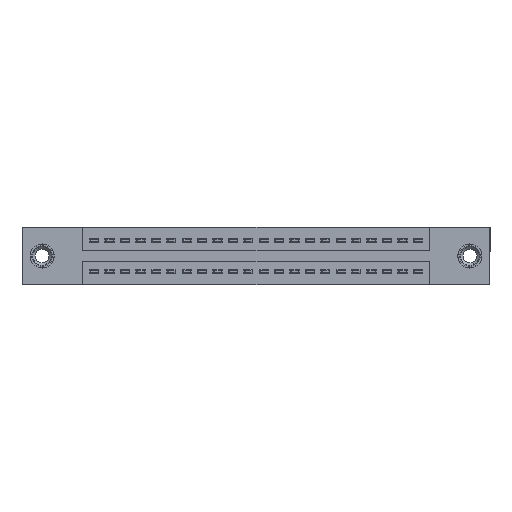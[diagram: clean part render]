
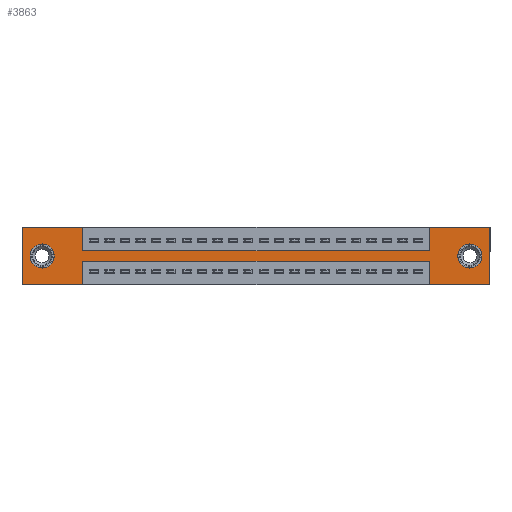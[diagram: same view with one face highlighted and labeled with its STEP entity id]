
A CAD part, front view. The second image highlights one B-rep face of the part: STEP entity #3863.
In plain terms, the highlighted planar face has unit normal (0, -1, 0).
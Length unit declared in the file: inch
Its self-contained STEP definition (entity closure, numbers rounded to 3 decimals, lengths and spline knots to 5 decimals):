
#450 = ORIENTED_EDGE ( 'NONE', *, *, #12869, .T. ) ;
#451 = DIRECTION ( 'NONE',  ( 0., 0., 1. ) ) ;
#697 = DIRECTION ( 'NONE',  ( 0., 0., -1. ) ) ;
#717 = AXIS2_PLACEMENT_3D ( 'NONE', #17985, #14445, #5999 ) ;
#838 = EDGE_CURVE ( 'NONE', #7861, #16075, #21256, .T. ) ;
#957 = DIRECTION ( 'NONE',  ( 1., 0., 0. ) ) ;
#1000 = EDGE_CURVE ( 'NONE', #19194, #17396, #4500, .T. ) ;
#1009 = LINE ( 'NONE', #6715, #16148 ) ;
#1046 = AXIS2_PLACEMENT_3D ( 'NONE', #6978, #21012, #697 ) ;
#1279 = VECTOR ( 'NONE', #3150, 39.37008 ) ;
#1291 = CARTESIAN_POINT ( 'NONE',  ( 2.6425, 0., 0. ) ) ;
#1867 = VERTEX_POINT ( 'NONE', #8113 ) ;
#2496 = EDGE_CURVE ( 'NONE', #21673, #8818, #1009, .T. ) ;
#2686 = DIRECTION ( 'NONE',  ( 0., 0., 1. ) ) ;
#2792 = VERTEX_POINT ( 'NONE', #11082 ) ;
#2934 = CARTESIAN_POINT ( 'NONE',  ( 0., 0., 0. ) ) ;
#2990 = CARTESIAN_POINT ( 'NONE',  ( 0.3925, 0., -0.22 ) ) ;
#3042 = DIRECTION ( 'NONE',  ( 0., 1., 0. ) ) ;
#3150 = DIRECTION ( 'NONE',  ( 1., 0., 0. ) ) ;
#3198 = VECTOR ( 'NONE', #8147, 39.37008 ) ;
#3420 = VERTEX_POINT ( 'NONE', #20329 ) ;
#3492 = VERTEX_POINT ( 'NONE', #18087 ) ;
#3514 = ORIENTED_EDGE ( 'NONE', *, *, #14309, .F. ) ;
#3753 = CARTESIAN_POINT ( 'NONE',  ( 0.13, 0., -0.185 ) ) ;
#3807 = CARTESIAN_POINT ( 'NONE',  ( 0., 0., -0.37 ) ) ;
#3863 = ADVANCED_FACE ( 'NONE', ( #10494, #9686, #5948 ), #14622, .T. ) ;
#4062 = VERTEX_POINT ( 'NONE', #17264 ) ;
#4108 = EDGE_CURVE ( 'NONE', #17717, #3492, #16592, .T. ) ;
#4135 = LINE ( 'NONE', #7260, #18784 ) ;
#4254 = DIRECTION ( 'NONE',  ( 0., 0., 1. ) ) ;
#4474 = DIRECTION ( 'NONE',  ( 0., 0., -1. ) ) ;
#4500 = LINE ( 'NONE', #1291, #3198 ) ;
#5116 = ORIENTED_EDGE ( 'NONE', *, *, #6029, .F. ) ;
#5344 = ORIENTED_EDGE ( 'NONE', *, *, #2496, .F. ) ;
#5537 = ORIENTED_EDGE ( 'NONE', *, *, #838, .F. ) ;
#5947 = VECTOR ( 'NONE', #4254, 39.37008 ) ;
#5948 = FACE_OUTER_BOUND ( 'NONE', #17070, .T. ) ;
#5999 = DIRECTION ( 'NONE',  ( 0., 0., 1. ) ) ;
#6029 = EDGE_CURVE ( 'NONE', #18850, #2792, #16251, .T. ) ;
#6118 = DIRECTION ( 'NONE',  ( 0., -1., 0. ) ) ;
#6328 = VECTOR ( 'NONE', #8868, 39.37008 ) ;
#6452 = DIRECTION ( 'NONE',  ( 0., 0., -1. ) ) ;
#6715 = CARTESIAN_POINT ( 'NONE',  ( 0.3925, 0., -0.22 ) ) ;
#6872 = EDGE_CURVE ( 'NONE', #15528, #1867, #12250, .T. ) ;
#6967 = DIRECTION ( 'NONE',  ( 0., 0., -1. ) ) ;
#6978 = CARTESIAN_POINT ( 'NONE',  ( 2.905, 0., -0.185 ) ) ;
#7174 = CARTESIAN_POINT ( 'NONE',  ( 0.3925, 0., -0.15 ) ) ;
#7260 = CARTESIAN_POINT ( 'NONE',  ( 2.6425, 0., -0.37 ) ) ;
#7368 = LINE ( 'NONE', #17730, #6328 ) ;
#7513 = CARTESIAN_POINT ( 'NONE',  ( 0., 0., 0. ) ) ;
#7577 = CIRCLE ( 'NONE', #1046, 0.078 ) ;
#7738 = EDGE_CURVE ( 'NONE', #17396, #18850, #7368, .T. ) ;
#7777 = EDGE_LOOP ( 'NONE', ( #15441, #13255 ) ) ;
#7861 = VERTEX_POINT ( 'NONE', #15959 ) ;
#7995 = EDGE_CURVE ( 'NONE', #3420, #7861, #19632, .T. ) ;
#8113 = CARTESIAN_POINT ( 'NONE',  ( 0.13, 0., -0.107 ) ) ;
#8147 = DIRECTION ( 'NONE',  ( 0., 0., 1. ) ) ;
#8208 = VECTOR ( 'NONE', #10220, 39.37008 ) ;
#8230 = CARTESIAN_POINT ( 'NONE',  ( 2.6425, 0., 0. ) ) ;
#8436 = CARTESIAN_POINT ( 'NONE',  ( 2.905, 0., -0.263 ) ) ;
#8455 = DIRECTION ( 'NONE',  ( -1., 0., 0. ) ) ;
#8530 = ORIENTED_EDGE ( 'NONE', *, *, #7995, .F. ) ;
#8642 = VECTOR ( 'NONE', #12900, 39.37008 ) ;
#8693 = AXIS2_PLACEMENT_3D ( 'NONE', #3753, #15662, #451 ) ;
#8818 = VERTEX_POINT ( 'NONE', #2990 ) ;
#8868 = DIRECTION ( 'NONE',  ( 1., 0., 0. ) ) ;
#8980 = VERTEX_POINT ( 'NONE', #8436 ) ;
#9023 = VECTOR ( 'NONE', #6967, 39.37008 ) ;
#9129 = EDGE_CURVE ( 'NONE', #8818, #17717, #9462, .T. ) ;
#9171 = CARTESIAN_POINT ( 'NONE',  ( 2.905, 0., -0.107 ) ) ;
#9462 = LINE ( 'NONE', #19499, #8642 ) ;
#9533 = ORIENTED_EDGE ( 'NONE', *, *, #9129, .F. ) ;
#9686 = FACE_BOUND ( 'NONE', #14235, .T. ) ;
#10138 = CARTESIAN_POINT ( 'NONE',  ( 0.3925, 0., 0. ) ) ;
#10220 = DIRECTION ( 'NONE',  ( 0., 0., -1. ) ) ;
#10453 = ORIENTED_EDGE ( 'NONE', *, *, #4108, .F. ) ;
#10494 = FACE_BOUND ( 'NONE', #7777, .T. ) ;
#10948 = CARTESIAN_POINT ( 'NONE',  ( 0.3925, 0., -0.15 ) ) ;
#11082 = CARTESIAN_POINT ( 'NONE',  ( 3.035, 0., -0.37 ) ) ;
#11268 = ORIENTED_EDGE ( 'NONE', *, *, #7738, .F. ) ;
#11320 = CARTESIAN_POINT ( 'NONE',  ( 0., 0., -0.37 ) ) ;
#11463 = ORIENTED_EDGE ( 'NONE', *, *, #17639, .F. ) ;
#11595 = CARTESIAN_POINT ( 'NONE',  ( 0., 0., -0.37 ) ) ;
#12250 = CIRCLE ( 'NONE', #8693, 0.078 ) ;
#12554 = AXIS2_PLACEMENT_3D ( 'NONE', #11320, #6118, #4474 ) ;
#12603 = EDGE_CURVE ( 'NONE', #16075, #19194, #20177, .T. ) ;
#12869 = EDGE_CURVE ( 'NONE', #1867, #15528, #15147, .T. ) ;
#12900 = DIRECTION ( 'NONE',  ( 0., 0., -1. ) ) ;
#13239 = CARTESIAN_POINT ( 'NONE',  ( 2.905, 0., -0.185 ) ) ;
#13255 = ORIENTED_EDGE ( 'NONE', *, *, #16276, .T. ) ;
#14235 = EDGE_LOOP ( 'NONE', ( #450, #20713 ) ) ;
#14309 = EDGE_CURVE ( 'NONE', #4062, #21673, #4135, .T. ) ;
#14445 = DIRECTION ( 'NONE',  ( 0., 1., 0. ) ) ;
#14622 = PLANE ( 'NONE',  #12554 ) ;
#14946 = CARTESIAN_POINT ( 'NONE',  ( 3.035, 0., 0. ) ) ;
#15147 = CIRCLE ( 'NONE', #717, 0.078 ) ;
#15441 = ORIENTED_EDGE ( 'NONE', *, *, #16992, .T. ) ;
#15481 = CARTESIAN_POINT ( 'NONE',  ( 3.035, 0., 0. ) ) ;
#15528 = VERTEX_POINT ( 'NONE', #16933 ) ;
#15662 = DIRECTION ( 'NONE',  ( 0., 1., 0. ) ) ;
#15959 = CARTESIAN_POINT ( 'NONE',  ( 0.3925, 0., 0. ) ) ;
#16075 = VERTEX_POINT ( 'NONE', #7174 ) ;
#16148 = VECTOR ( 'NONE', #8455, 39.37008 ) ;
#16206 = VECTOR ( 'NONE', #957, 39.37008 ) ;
#16251 = LINE ( 'NONE', #15481, #9023 ) ;
#16276 = EDGE_CURVE ( 'NONE', #8980, #17974, #7577, .T. ) ;
#16384 = CIRCLE ( 'NONE', #21089, 0.078 ) ;
#16592 = LINE ( 'NONE', #3807, #19507 ) ;
#16864 = EDGE_CURVE ( 'NONE', #2792, #4062, #18242, .T. ) ;
#16933 = CARTESIAN_POINT ( 'NONE',  ( 0.13, 0., -0.263 ) ) ;
#16937 = DIRECTION ( 'NONE',  ( -1., 0., 0. ) ) ;
#16988 = CARTESIAN_POINT ( 'NONE',  ( 2.6425, 0., -0.15 ) ) ;
#16992 = EDGE_CURVE ( 'NONE', #17974, #8980, #16384, .T. ) ;
#17070 = EDGE_LOOP ( 'NONE', ( #9533, #5344, #3514, #20644, #5116, #11268, #20798, #19907, #5537, #8530, #11463, #10453 ) ) ;
#17264 = CARTESIAN_POINT ( 'NONE',  ( 2.6425, 0., -0.37 ) ) ;
#17396 = VERTEX_POINT ( 'NONE', #8230 ) ;
#17403 = LINE ( 'NONE', #7513, #5947 ) ;
#17494 = DIRECTION ( 'NONE',  ( -1., 0., 0. ) ) ;
#17639 = EDGE_CURVE ( 'NONE', #3492, #3420, #17403, .T. ) ;
#17717 = VERTEX_POINT ( 'NONE', #20216 ) ;
#17730 = CARTESIAN_POINT ( 'NONE',  ( 0., 0., 0. ) ) ;
#17974 = VERTEX_POINT ( 'NONE', #9171 ) ;
#17985 = CARTESIAN_POINT ( 'NONE',  ( 0.13, 0., -0.185 ) ) ;
#18087 = CARTESIAN_POINT ( 'NONE',  ( 0., 0., -0.37 ) ) ;
#18242 = LINE ( 'NONE', #11595, #19315 ) ;
#18663 = CARTESIAN_POINT ( 'NONE',  ( 2.6425, 0., -0.22 ) ) ;
#18784 = VECTOR ( 'NONE', #2686, 39.37008 ) ;
#18850 = VERTEX_POINT ( 'NONE', #14946 ) ;
#19194 = VERTEX_POINT ( 'NONE', #16988 ) ;
#19315 = VECTOR ( 'NONE', #16937, 39.37008 ) ;
#19499 = CARTESIAN_POINT ( 'NONE',  ( 0.3925, 0., -0.37 ) ) ;
#19507 = VECTOR ( 'NONE', #17494, 39.37008 ) ;
#19632 = LINE ( 'NONE', #2934, #1279 ) ;
#19907 = ORIENTED_EDGE ( 'NONE', *, *, #12603, .F. ) ;
#20177 = LINE ( 'NONE', #10948, #16206 ) ;
#20216 = CARTESIAN_POINT ( 'NONE',  ( 0.3925, 0., -0.37 ) ) ;
#20329 = CARTESIAN_POINT ( 'NONE',  ( 0., 0., 0. ) ) ;
#20644 = ORIENTED_EDGE ( 'NONE', *, *, #16864, .F. ) ;
#20713 = ORIENTED_EDGE ( 'NONE', *, *, #6872, .T. ) ;
#20798 = ORIENTED_EDGE ( 'NONE', *, *, #1000, .F. ) ;
#21012 = DIRECTION ( 'NONE',  ( 0., 1., 0. ) ) ;
#21089 = AXIS2_PLACEMENT_3D ( 'NONE', #13239, #3042, #6452 ) ;
#21256 = LINE ( 'NONE', #10138, #8208 ) ;
#21673 = VERTEX_POINT ( 'NONE', #18663 ) ;
